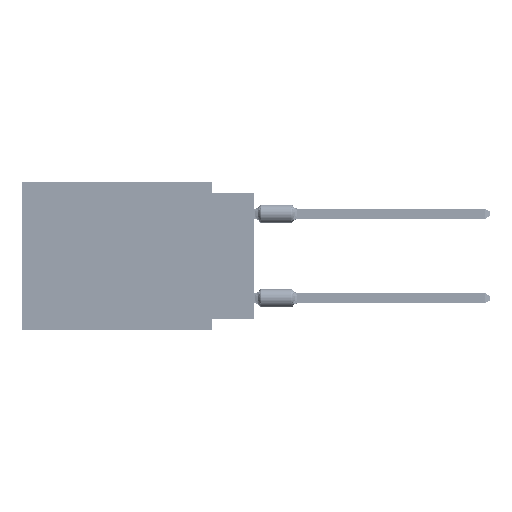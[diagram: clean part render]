
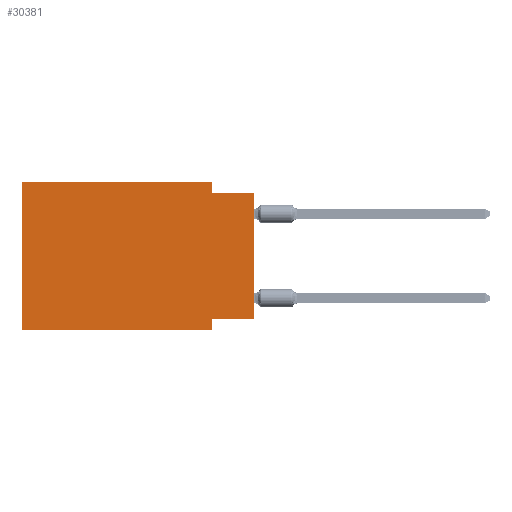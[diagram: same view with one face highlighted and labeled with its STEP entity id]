
A CAD part, left-side view. The second image highlights one B-rep face of the part: STEP entity #30381.
In plain terms, the highlighted planar face has unit normal (-1, 0, 0).
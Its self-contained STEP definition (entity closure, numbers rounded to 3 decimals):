
#747 = VERTEX_POINT ( 'NONE', #52166 ) ;
#2859 = VERTEX_POINT ( 'NONE', #102115 ) ;
#6261 = CARTESIAN_POINT ( 'NONE',  ( 0., 0., 0. ) ) ;
#6580 = LINE ( 'NONE', #61159, #88756 ) ;
#6693 = CARTESIAN_POINT ( 'NONE',  ( 0., 13.97, 0. ) ) ;
#9058 = ORIENTED_EDGE ( 'NONE', *, *, #10561, .F. ) ;
#9219 = VERTEX_POINT ( 'NONE', #111703 ) ;
#10561 = EDGE_CURVE ( 'NONE', #60595, #93286, #92677, .T. ) ;
#11128 = EDGE_CURVE ( 'NONE', #53447, #43247, #102721, .T. ) ;
#12062 = VECTOR ( 'NONE', #27289, 1000. ) ;
#14845 = CARTESIAN_POINT ( 'NONE',  ( 0., 2.54, -8.89 ) ) ;
#15684 = DIRECTION ( 'NONE',  ( 0., 0., -1. ) ) ;
#15764 = ORIENTED_EDGE ( 'NONE', *, *, #39043, .T. ) ;
#19525 = CARTESIAN_POINT ( 'NONE',  ( 0., 13.97, 0. ) ) ;
#25161 = ORIENTED_EDGE ( 'NONE', *, *, #11128, .F. ) ;
#25535 = EDGE_CURVE ( 'NONE', #53447, #747, #106459, .T. ) ;
#27263 = LINE ( 'NONE', #14845, #52560 ) ;
#27289 = DIRECTION ( 'NONE',  ( 0., -1., 0. ) ) ;
#29947 = DIRECTION ( 'NONE',  ( 0., -1., 0. ) ) ;
#30381 = ADVANCED_FACE ( 'NONE', ( #79892 ), #32488, .F. ) ;
#31206 = VECTOR ( 'NONE', #29947, 1000. ) ;
#31313 = CARTESIAN_POINT ( 'NONE',  ( 0., 2.54, -8.255 ) ) ;
#32488 = PLANE ( 'NONE',  #62364 ) ;
#36599 = EDGE_CURVE ( 'NONE', #39279, #747, #104307, .T. ) ;
#37459 = ORIENTED_EDGE ( 'NONE', *, *, #103557, .F. ) ;
#37934 = ORIENTED_EDGE ( 'NONE', *, *, #98795, .F. ) ;
#39043 = EDGE_CURVE ( 'NONE', #2859, #9219, #6580, .T. ) ;
#39279 = VERTEX_POINT ( 'NONE', #86518 ) ;
#40256 = CARTESIAN_POINT ( 'NONE',  ( 0., 0., -8.255 ) ) ;
#43247 = VERTEX_POINT ( 'NONE', #31313 ) ;
#51743 = ORIENTED_EDGE ( 'NONE', *, *, #63439, .F. ) ;
#52166 = CARTESIAN_POINT ( 'NONE',  ( 0., 0., -0.635 ) ) ;
#52560 = VECTOR ( 'NONE', #69460, 1000. ) ;
#52882 = DIRECTION ( 'NONE',  ( 1., 0., 0. ) ) ;
#53447 = VERTEX_POINT ( 'NONE', #64500 ) ;
#57506 = CARTESIAN_POINT ( 'NONE',  ( 0., 2.54, 0. ) ) ;
#60595 = VERTEX_POINT ( 'NONE', #104919 ) ;
#61159 = CARTESIAN_POINT ( 'NONE',  ( 0., 13.97, -8.89 ) ) ;
#62364 = AXIS2_PLACEMENT_3D ( 'NONE', #6693, #52882, #15684 ) ;
#63348 = DIRECTION ( 'NONE',  ( 0., 0., 1. ) ) ;
#63439 = EDGE_CURVE ( 'NONE', #93286, #39279, #112147, .T. ) ;
#64500 = CARTESIAN_POINT ( 'NONE',  ( 0., 0., -8.255 ) ) ;
#69460 = DIRECTION ( 'NONE',  ( 0., 0., -1. ) ) ;
#77307 = CARTESIAN_POINT ( 'NONE',  ( 0., 0., -0.635 ) ) ;
#79892 = FACE_OUTER_BOUND ( 'NONE', #94529, .T. ) ;
#80965 = DIRECTION ( 'NONE',  ( 0., -1., 0. ) ) ;
#84473 = VECTOR ( 'NONE', #96265, 1000. ) ;
#86518 = CARTESIAN_POINT ( 'NONE',  ( 0., 2.54, -0.635 ) ) ;
#88756 = VECTOR ( 'NONE', #80965, 1000. ) ;
#90693 = VECTOR ( 'NONE', #115086, 1000. ) ;
#92677 = LINE ( 'NONE', #109476, #12062 ) ;
#93286 = VERTEX_POINT ( 'NONE', #98199 ) ;
#94116 = DIRECTION ( 'NONE',  ( 0., 0., -1. ) ) ;
#94529 = EDGE_LOOP ( 'NONE', ( #104057, #105808, #51743, #9058, #37934, #15764, #37459, #25161 ) ) ;
#96265 = DIRECTION ( 'NONE',  ( 0., 0., 1. ) ) ;
#98199 = CARTESIAN_POINT ( 'NONE',  ( 0., 2.54, 0. ) ) ;
#98795 = EDGE_CURVE ( 'NONE', #2859, #60595, #108949, .T. ) ;
#102115 = CARTESIAN_POINT ( 'NONE',  ( 0., 13.97, -8.89 ) ) ;
#102721 = LINE ( 'NONE', #40256, #90693 ) ;
#103023 = VECTOR ( 'NONE', #94116, 1000. ) ;
#103557 = EDGE_CURVE ( 'NONE', #43247, #9219, #27263, .T. ) ;
#104057 = ORIENTED_EDGE ( 'NONE', *, *, #25535, .T. ) ;
#104307 = LINE ( 'NONE', #77307, #31206 ) ;
#104919 = CARTESIAN_POINT ( 'NONE',  ( 0., 13.97, 0. ) ) ;
#105808 = ORIENTED_EDGE ( 'NONE', *, *, #36599, .F. ) ;
#106459 = LINE ( 'NONE', #6261, #84473 ) ;
#108949 = LINE ( 'NONE', #19525, #113387 ) ;
#109476 = CARTESIAN_POINT ( 'NONE',  ( 0., 13.97, 0. ) ) ;
#111703 = CARTESIAN_POINT ( 'NONE',  ( 0., 2.54, -8.89 ) ) ;
#112147 = LINE ( 'NONE', #57506, #103023 ) ;
#113387 = VECTOR ( 'NONE', #63348, 1000. ) ;
#115086 = DIRECTION ( 'NONE',  ( 0., 1., 0. ) ) ;
